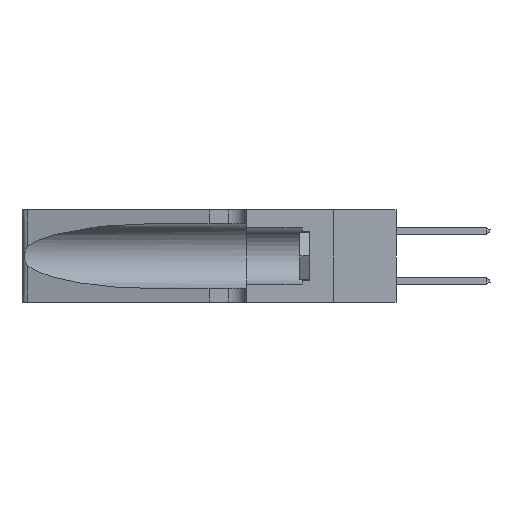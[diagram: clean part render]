
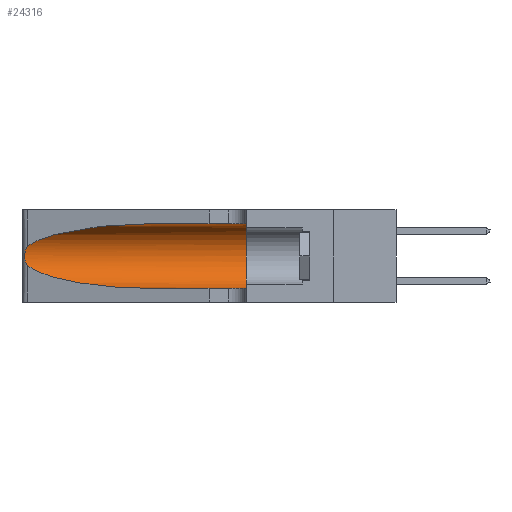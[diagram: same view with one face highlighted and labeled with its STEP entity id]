
A CAD part, left-side view. The second image highlights one B-rep face of the part: STEP entity #24316.
In plain terms, the highlighted cylindrical face has radius 3.308 mm (diameter 6.617 mm), a partial arc.
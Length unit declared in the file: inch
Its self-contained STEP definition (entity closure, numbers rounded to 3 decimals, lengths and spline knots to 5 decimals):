
#864 = CIRCLE ( 'NONE', #1900, 0.13025 ) ;
#1607 = ORIENTED_EDGE ( 'NONE', *, *, #29011, .T. ) ;
#1631 = EDGE_LOOP ( 'NONE', ( #37130, #1607, #34069, #18454, #7114, #40956 ) ) ;
#1900 = AXIS2_PLACEMENT_3D ( 'NONE', #15951, #38691, #19275 ) ;
#2510 = CARTESIAN_POINT ( 'NONE',  ( 0.26075, 1.23896, 0.19203 ) ) ;
#3707 =( BOUNDED_CURVE ( )  B_SPLINE_CURVE ( 3, ( #33396, #4006, #39922, #20482 ),
 .UNSPECIFIED., .F., .F. ) 
 B_SPLINE_CURVE_WITH_KNOTS ( ( 4, 4 ),
 ( 1.5708, 2.84003 ),
 .UNSPECIFIED. ) 
 CURVE ( )  GEOMETRIC_REPRESENTATION_ITEM ( )  RATIONAL_B_SPLINE_CURVE ( ( 1., 0.87, 0.87, 1. ) ) 
 REPRESENTATION_ITEM ( '' )  );
#4006 = CARTESIAN_POINT ( 'NONE',  ( 0.18966, 0.96281, 0.31525 ) ) ;
#4190 = VERTEX_POINT ( 'NONE', #35767 ) ;
#4579 = VERTEX_POINT ( 'NONE', #5105 ) ;
#5105 = CARTESIAN_POINT ( 'NONE',  ( 0.1305, 0.35, 0.05475 ) ) ;
#5716 = CARTESIAN_POINT ( 'NONE',  ( 0.25487, 1.22718, 0.22369 ) ) ;
#5858 = CARTESIAN_POINT ( 'NONE',  ( 0.26017, 1.23833, 0.17102 ) ) ;
#7114 = ORIENTED_EDGE ( 'NONE', *, *, #33276, .F. ) ;
#9150 = CARTESIAN_POINT ( 'NONE',  ( 0.25789, 1.23486, 0.15765 ) ) ;
#9722 = CARTESIAN_POINT ( 'NONE',  ( 0.1305, 0.35, 0.31525 ) ) ;
#11259 = CARTESIAN_POINT ( 'NONE',  ( 0.2373, 1.15595, 0.08982 ) ) ;
#11350 =( BOUNDED_CURVE ( )  B_SPLINE_CURVE ( 3, ( #33907, #11259, #14571, #37298 ),
 .UNSPECIFIED., .F., .F. ) 
 B_SPLINE_CURVE_WITH_KNOTS ( ( 4, 4 ),
 ( 3.44316, 4.71239 ),
 .UNSPECIFIED. ) 
 CURVE ( )  GEOMETRIC_REPRESENTATION_ITEM ( )  RATIONAL_B_SPLINE_CURVE ( ( 1., 0.87, 0.87, 1. ) ) 
 REPRESENTATION_ITEM ( '' )  );
#12418 = CARTESIAN_POINT ( 'NONE',  ( 0.25555, 1.22993, 0.14849 ) ) ;
#12713 = CARTESIAN_POINT ( 'NONE',  ( 0.25487, 1.22718, 0.14631 ) ) ;
#13184 = VERTEX_POINT ( 'NONE', #9722 ) ;
#13885 = LINE ( 'NONE', #32674, #28134 ) ;
#14540 = CARTESIAN_POINT ( 'NONE',  ( 0.25487, 1.22718, 0.22369 ) ) ;
#14571 = CARTESIAN_POINT ( 'NONE',  ( 0.18966, 0.96281, 0.05475 ) ) ;
#15951 = CARTESIAN_POINT ( 'NONE',  ( 0.1305, 0.35, 0.185 ) ) ;
#16323 = DIRECTION ( 'NONE',  ( 0., 0., -1. ) ) ;
#17060 = EDGE_CURVE ( 'NONE', #27123, #4579, #13885, .T. ) ;
#17296 = DIRECTION ( 'NONE',  ( 0., -1., 0. ) ) ;
#17554 = VERTEX_POINT ( 'NONE', #12713 ) ;
#18454 = ORIENTED_EDGE ( 'NONE', *, *, #17060, .T. ) ;
#18779 = CARTESIAN_POINT ( 'NONE',  ( 0.25555, 1.22994, 0.2215 ) ) ;
#18910 = CARTESIAN_POINT ( 'NONE',  ( 0.25787, 1.23484, 0.2124 ) ) ;
#19275 = DIRECTION ( 'NONE',  ( 0., 0., 1. ) ) ;
#19451 = EDGE_CURVE ( 'NONE', #17554, #27123, #11350, .T. ) ;
#20482 = CARTESIAN_POINT ( 'NONE',  ( 0.25487, 1.22718, 0.22369 ) ) ;
#21853 = EDGE_CURVE ( 'NONE', #4190, #37230, #3707, .T. ) ;
#22152 = CARTESIAN_POINT ( 'NONE',  ( 0.26018, 1.23835, 0.19895 ) ) ;
#22886 = CARTESIAN_POINT ( 'NONE',  ( 0.1305, 1.61858, 0.185 ) ) ;
#24316 = ADVANCED_FACE ( 'NONE', ( #38518 ), #28858, .F. ) ;
#25410 = CARTESIAN_POINT ( 'NONE',  ( 0.26075, 1.23896, 0.178 ) ) ;
#26124 = DIRECTION ( 'NONE',  ( 0., -1., 0. ) ) ;
#27123 = VERTEX_POINT ( 'NONE', #36195 ) ;
#27217 = EDGE_CURVE ( 'NONE', #4190, #13184, #34271, .T. ) ;
#28134 = VECTOR ( 'NONE', #39120, 39.37008 ) ;
#28672 = CARTESIAN_POINT ( 'NONE',  ( 0.25856, 1.23593, 0.16098 ) ) ;
#28858 = CYLINDRICAL_SURFACE ( 'NONE', #41460, 0.13025 ) ;
#29011 = EDGE_CURVE ( 'NONE', #37230, #17554, #38483, .T. ) ;
#31944 = CARTESIAN_POINT ( 'NONE',  ( 0.25639, 1.23186, 0.15144 ) ) ;
#32674 = CARTESIAN_POINT ( 'NONE',  ( 0.1305, 1.61858, 0.05475 ) ) ;
#33276 = EDGE_CURVE ( 'NONE', #13184, #4579, #864, .T. ) ;
#33396 = CARTESIAN_POINT ( 'NONE',  ( 0.1305, 0.72297, 0.31525 ) ) ;
#33907 = CARTESIAN_POINT ( 'NONE',  ( 0.25487, 1.22718, 0.14631 ) ) ;
#34069 = ORIENTED_EDGE ( 'NONE', *, *, #19451, .T. ) ;
#34271 = LINE ( 'NONE', #40010, #41883 ) ;
#35212 = CARTESIAN_POINT ( 'NONE',  ( 0.25487, 1.22718, 0.14631 ) ) ;
#35767 = CARTESIAN_POINT ( 'NONE',  ( 0.1305, 0.72297, 0.31525 ) ) ;
#36195 = CARTESIAN_POINT ( 'NONE',  ( 0.1305, 0.72297, 0.05475 ) ) ;
#37130 = ORIENTED_EDGE ( 'NONE', *, *, #21853, .T. ) ;
#37230 = VERTEX_POINT ( 'NONE', #14540 ) ;
#37298 = CARTESIAN_POINT ( 'NONE',  ( 0.1305, 0.72297, 0.05475 ) ) ;
#38321 = CARTESIAN_POINT ( 'NONE',  ( 0.25639, 1.23184, 0.21858 ) ) ;
#38483 = B_SPLINE_CURVE_WITH_KNOTS ( 'NONE', 3,
 ( #5716, #18779, #38321, #18910, #41586, #22152, #2510, #25410, #5858, #28672, #9150, #31944, #12418, #35212 ),
 .UNSPECIFIED., .F., .F.,
 ( 4, 2, 2, 2, 2, 2, 4 ),
 ( 0., 0.00027, 0.00053, 0.00107, 0.0016, 0.00187, 0.00214 ),
 .UNSPECIFIED. ) ;
#38518 = FACE_OUTER_BOUND ( 'NONE', #1631, .T. ) ;
#38691 = DIRECTION ( 'NONE',  ( 0., 1., 0. ) ) ;
#39120 = DIRECTION ( 'NONE',  ( 0., -1., 0. ) ) ;
#39922 = CARTESIAN_POINT ( 'NONE',  ( 0.2373, 1.15595, 0.28018 ) ) ;
#40010 = CARTESIAN_POINT ( 'NONE',  ( 0.1305, 1.61858, 0.31525 ) ) ;
#40956 = ORIENTED_EDGE ( 'NONE', *, *, #27217, .F. ) ;
#41460 = AXIS2_PLACEMENT_3D ( 'NONE', #22886, #26124, #16323 ) ;
#41586 = CARTESIAN_POINT ( 'NONE',  ( 0.25854, 1.2359, 0.20912 ) ) ;
#41883 = VECTOR ( 'NONE', #17296, 39.37008 ) ;
